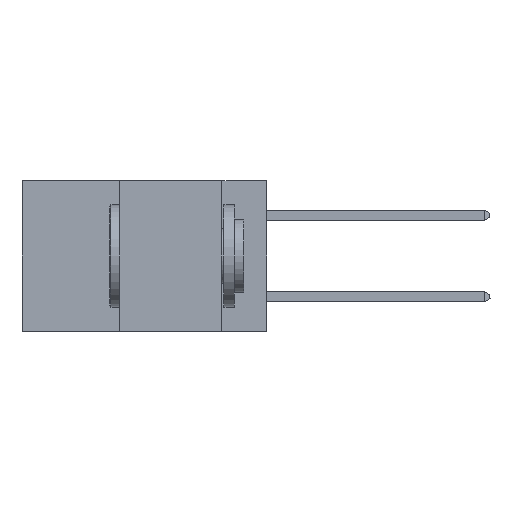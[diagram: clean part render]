
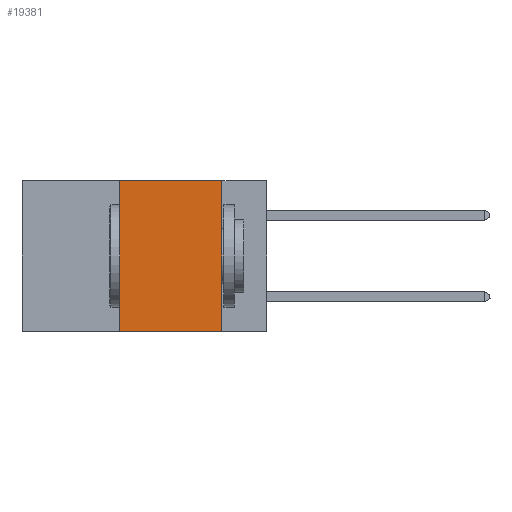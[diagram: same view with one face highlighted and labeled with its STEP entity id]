
A CAD part, left-side view. The second image highlights one B-rep face of the part: STEP entity #19381.
In plain terms, the highlighted planar face has unit normal (-1, 0, 0).
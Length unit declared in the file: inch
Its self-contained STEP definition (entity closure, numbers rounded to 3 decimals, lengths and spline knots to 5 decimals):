
#880 = FACE_OUTER_BOUND ( 'NONE', #14040, .T. ) ;
#1856 = PLANE ( 'NONE',  #19469 ) ;
#2736 = LINE ( 'NONE', #13318, #6409 ) ;
#3433 = DIRECTION ( 'NONE',  ( 1., 0., 0. ) ) ;
#4508 = CARTESIAN_POINT ( 'NONE',  ( 0., 0.11, 0. ) ) ;
#4811 = CARTESIAN_POINT ( 'NONE',  ( 0., 0.36, 0. ) ) ;
#5277 = VERTEX_POINT ( 'NONE', #19031 ) ;
#5676 = DIRECTION ( 'NONE',  ( 0., -1., 0. ) ) ;
#5819 = CARTESIAN_POINT ( 'NONE',  ( 0., 0.36, -0.37 ) ) ;
#6409 = VECTOR ( 'NONE', #5676, 39.37008 ) ;
#6443 = VECTOR ( 'NONE', #15495, 39.37008 ) ;
#6750 = VECTOR ( 'NONE', #14104, 39.37008 ) ;
#6800 = EDGE_CURVE ( 'NONE', #10573, #16878, #2736, .T. ) ;
#6841 = DIRECTION ( 'NONE',  ( 0., 0., -1. ) ) ;
#7237 = ORIENTED_EDGE ( 'NONE', *, *, #7725, .T. ) ;
#7359 = ORIENTED_EDGE ( 'NONE', *, *, #6800, .F. ) ;
#7572 = CARTESIAN_POINT ( 'NONE',  ( 0., 0.6, -0.37 ) ) ;
#7725 = EDGE_CURVE ( 'NONE', #15624, #5277, #13803, .T. ) ;
#8627 = CARTESIAN_POINT ( 'NONE',  ( 0., 0.11, 0. ) ) ;
#9143 = VECTOR ( 'NONE', #20090, 39.37008 ) ;
#10573 = VERTEX_POINT ( 'NONE', #14686 ) ;
#10882 = LINE ( 'NONE', #4811, #6443 ) ;
#10931 = LINE ( 'NONE', #4508, #6750 ) ;
#12428 = ORIENTED_EDGE ( 'NONE', *, *, #14989, .F. ) ;
#13065 = CARTESIAN_POINT ( 'NONE',  ( 0., 0.6, 0. ) ) ;
#13274 = EDGE_CURVE ( 'NONE', #16878, #5277, #10931, .T. ) ;
#13318 = CARTESIAN_POINT ( 'NONE',  ( 0., 0.6, 0. ) ) ;
#13803 = LINE ( 'NONE', #7572, #9143 ) ;
#14040 = EDGE_LOOP ( 'NONE', ( #18081, #7359, #12428, #7237 ) ) ;
#14104 = DIRECTION ( 'NONE',  ( 0., 0., -1. ) ) ;
#14686 = CARTESIAN_POINT ( 'NONE',  ( 0., 0.36, 0. ) ) ;
#14989 = EDGE_CURVE ( 'NONE', #15624, #10573, #10882, .T. ) ;
#15495 = DIRECTION ( 'NONE',  ( 0., 0., 1. ) ) ;
#15624 = VERTEX_POINT ( 'NONE', #5819 ) ;
#16878 = VERTEX_POINT ( 'NONE', #8627 ) ;
#18081 = ORIENTED_EDGE ( 'NONE', *, *, #13274, .F. ) ;
#19031 = CARTESIAN_POINT ( 'NONE',  ( 0., 0.11, -0.37 ) ) ;
#19381 = ADVANCED_FACE ( 'NONE', ( #880 ), #1856, .F. ) ;
#19469 = AXIS2_PLACEMENT_3D ( 'NONE', #13065, #3433, #6841 ) ;
#20090 = DIRECTION ( 'NONE',  ( 0., -1., 0. ) ) ;
